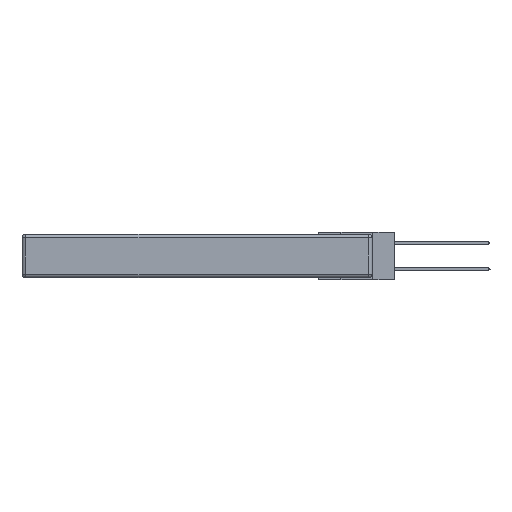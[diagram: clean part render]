
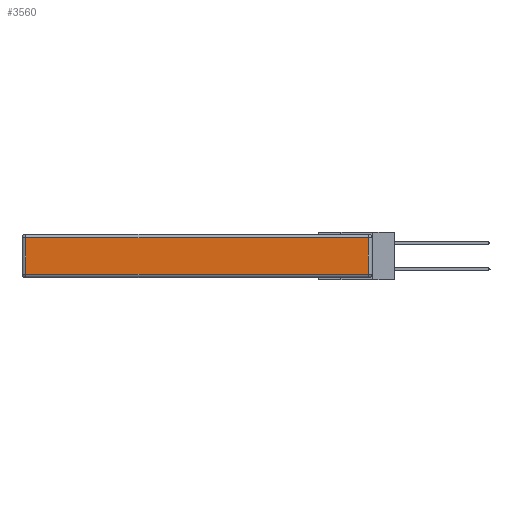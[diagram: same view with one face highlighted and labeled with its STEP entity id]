
A CAD part, left-side view. The second image highlights one B-rep face of the part: STEP entity #3560.
In plain terms, the highlighted planar face has unit normal (-1, 0, 0).
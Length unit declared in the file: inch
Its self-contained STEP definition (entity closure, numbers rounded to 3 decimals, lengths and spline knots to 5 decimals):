
#679 = EDGE_CURVE ( 'NONE', #1011, #16582, #13072, .T. ) ;
#866 = VECTOR ( 'NONE', #6848, 39.37008 ) ;
#1011 = VERTEX_POINT ( 'NONE', #9056 ) ;
#1346 = VECTOR ( 'NONE', #16238, 39.37008 ) ;
#1369 = CARTESIAN_POINT ( 'NONE',  ( 0., 2.72, -0.313 ) ) ;
#2582 = VECTOR ( 'NONE', #6420, 39.37008 ) ;
#3560 = ADVANCED_FACE ( 'NONE', ( #8572 ), #13342, .T. ) ;
#3580 = ORIENTED_EDGE ( 'NONE', *, *, #12439, .T. ) ;
#3659 = CARTESIAN_POINT ( 'NONE',  ( 0., 0.03, -0.343 ) ) ;
#4153 = CARTESIAN_POINT ( 'NONE',  ( 0., 0., -0.313 ) ) ;
#4828 = LINE ( 'NONE', #3659, #7113 ) ;
#5298 = DIRECTION ( 'NONE',  ( -1., 0., 0. ) ) ;
#5666 = DIRECTION ( 'NONE',  ( 0., 0., 1. ) ) ;
#6160 = LINE ( 'NONE', #10896, #1346 ) ;
#6353 = EDGE_LOOP ( 'NONE', ( #3580, #16964, #16976, #13603 ) ) ;
#6420 = DIRECTION ( 'NONE',  ( 0., 0., -1. ) ) ;
#6848 = DIRECTION ( 'NONE',  ( 0., -1., 0. ) ) ;
#7003 = CARTESIAN_POINT ( 'NONE',  ( 0., 0.03, -0.03 ) ) ;
#7113 = VECTOR ( 'NONE', #5666, 39.37008 ) ;
#7352 = EDGE_CURVE ( 'NONE', #13400, #1011, #6160, .T. ) ;
#8261 = CARTESIAN_POINT ( 'NONE',  ( 0., 2.72, -0.343 ) ) ;
#8572 = FACE_OUTER_BOUND ( 'NONE', #6353, .T. ) ;
#8715 = CARTESIAN_POINT ( 'NONE',  ( 0., 0.03, -0.313 ) ) ;
#9056 = CARTESIAN_POINT ( 'NONE',  ( 0., 2.72, -0.03 ) ) ;
#10896 = CARTESIAN_POINT ( 'NONE',  ( 0., 2.75, -0.03 ) ) ;
#11746 = EDGE_CURVE ( 'NONE', #14355, #13400, #4828, .T. ) ;
#11921 = AXIS2_PLACEMENT_3D ( 'NONE', #15961, #5298, #11927 ) ;
#11927 = DIRECTION ( 'NONE',  ( 0., 0., 1. ) ) ;
#12439 = EDGE_CURVE ( 'NONE', #16582, #14355, #13609, .T. ) ;
#13072 = LINE ( 'NONE', #8261, #2582 ) ;
#13342 = PLANE ( 'NONE',  #11921 ) ;
#13400 = VERTEX_POINT ( 'NONE', #7003 ) ;
#13603 = ORIENTED_EDGE ( 'NONE', *, *, #679, .T. ) ;
#13609 = LINE ( 'NONE', #4153, #866 ) ;
#14355 = VERTEX_POINT ( 'NONE', #8715 ) ;
#15961 = CARTESIAN_POINT ( 'NONE',  ( 0., 0., -0.343 ) ) ;
#16238 = DIRECTION ( 'NONE',  ( 0., 1., 0. ) ) ;
#16582 = VERTEX_POINT ( 'NONE', #1369 ) ;
#16964 = ORIENTED_EDGE ( 'NONE', *, *, #11746, .T. ) ;
#16976 = ORIENTED_EDGE ( 'NONE', *, *, #7352, .T. ) ;
